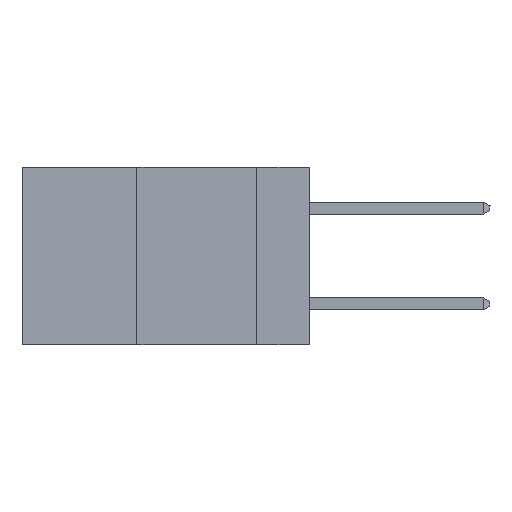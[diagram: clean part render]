
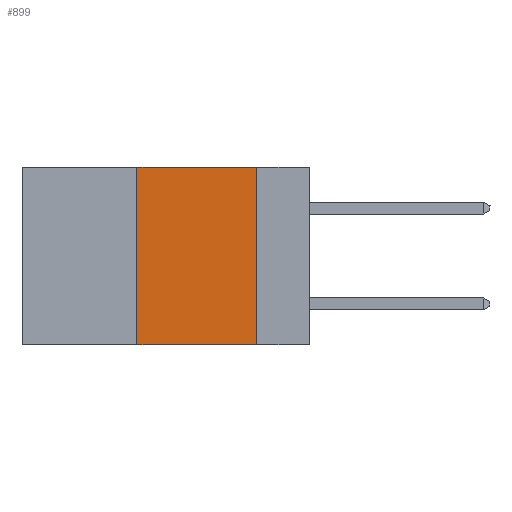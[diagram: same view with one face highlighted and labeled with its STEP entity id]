
A CAD part, left-side view. The second image highlights one B-rep face of the part: STEP entity #899.
In plain terms, the highlighted planar face has unit normal (-1, 0, 0).
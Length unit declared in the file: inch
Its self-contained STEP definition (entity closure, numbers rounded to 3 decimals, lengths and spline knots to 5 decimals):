
#175 = DIRECTION ( 'NONE',  ( 0., 0., -1. ) ) ;
#289 = VERTEX_POINT ( 'NONE', #15448 ) ;
#338 = ORIENTED_EDGE ( 'NONE', *, *, #414, .F. ) ;
#357 = VERTEX_POINT ( 'NONE', #15373 ) ;
#414 = EDGE_CURVE ( 'NONE', #6756, #357, #6771, .T. ) ;
#899 = ADVANCED_FACE ( 'NONE', ( #16993 ), #15452, .F. ) ;
#1769 = LINE ( 'NONE', #17431, #2991 ) ;
#2991 = VECTOR ( 'NONE', #4927, 39.37008 ) ;
#3026 = CARTESIAN_POINT ( 'NONE',  ( 0., 0.6, -0.37 ) ) ;
#3670 = VECTOR ( 'NONE', #12188, 39.37008 ) ;
#4927 = DIRECTION ( 'NONE',  ( 0., 0., -1. ) ) ;
#5200 = ORIENTED_EDGE ( 'NONE', *, *, #7180, .T. ) ;
#6089 = EDGE_CURVE ( 'NONE', #357, #289, #1769, .T. ) ;
#6122 = CARTESIAN_POINT ( 'NONE',  ( 0., 0.6, 0. ) ) ;
#6204 = EDGE_CURVE ( 'NONE', #11718, #6756, #13193, .T. ) ;
#6240 = CARTESIAN_POINT ( 'NONE',  ( 0., 0.36, 0. ) ) ;
#6756 = VERTEX_POINT ( 'NONE', #6240 ) ;
#6771 = LINE ( 'NONE', #9408, #14824 ) ;
#7180 = EDGE_CURVE ( 'NONE', #11718, #289, #15879, .T. ) ;
#8451 = ORIENTED_EDGE ( 'NONE', *, *, #6089, .F. ) ;
#9408 = CARTESIAN_POINT ( 'NONE',  ( 0., 0.6, 0. ) ) ;
#11718 = VERTEX_POINT ( 'NONE', #12393 ) ;
#12188 = DIRECTION ( 'NONE',  ( 0., -1., 0. ) ) ;
#12393 = CARTESIAN_POINT ( 'NONE',  ( 0., 0.36, -0.37 ) ) ;
#13063 = DIRECTION ( 'NONE',  ( 0., 0., 1. ) ) ;
#13193 = LINE ( 'NONE', #18170, #13956 ) ;
#13956 = VECTOR ( 'NONE', #13063, 39.37008 ) ;
#14824 = VECTOR ( 'NONE', #18802, 39.37008 ) ;
#15373 = CARTESIAN_POINT ( 'NONE',  ( 0., 0.11, 0. ) ) ;
#15448 = CARTESIAN_POINT ( 'NONE',  ( 0., 0.11, -0.37 ) ) ;
#15452 = PLANE ( 'NONE',  #18003 ) ;
#15879 = LINE ( 'NONE', #3026, #3670 ) ;
#16993 = FACE_OUTER_BOUND ( 'NONE', #17624, .T. ) ;
#17431 = CARTESIAN_POINT ( 'NONE',  ( 0., 0.11, 0. ) ) ;
#17624 = EDGE_LOOP ( 'NONE', ( #8451, #338, #17709, #5200 ) ) ;
#17709 = ORIENTED_EDGE ( 'NONE', *, *, #6204, .F. ) ;
#18003 = AXIS2_PLACEMENT_3D ( 'NONE', #6122, #18781, #175 ) ;
#18170 = CARTESIAN_POINT ( 'NONE',  ( 0., 0.36, 0. ) ) ;
#18781 = DIRECTION ( 'NONE',  ( 1., 0., 0. ) ) ;
#18802 = DIRECTION ( 'NONE',  ( 0., -1., 0. ) ) ;
